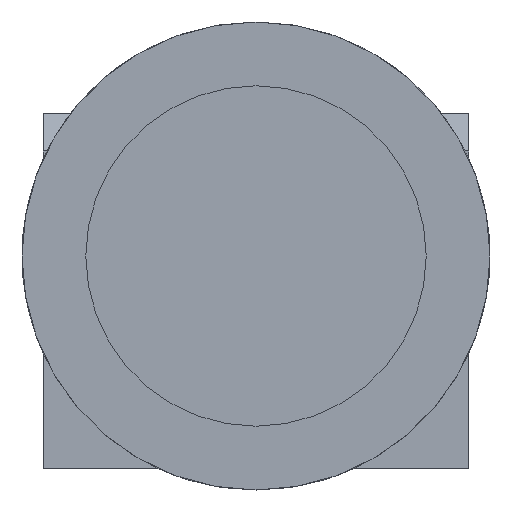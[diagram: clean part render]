
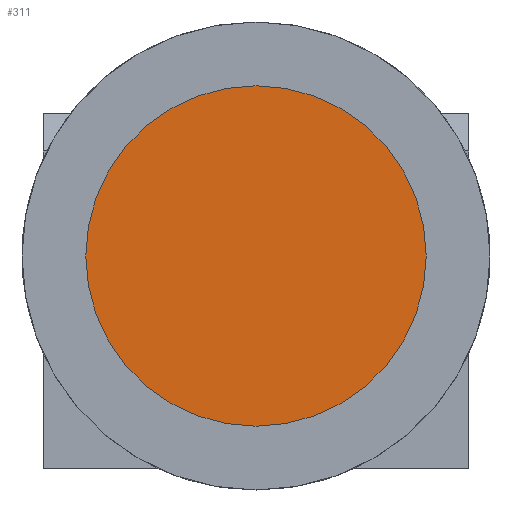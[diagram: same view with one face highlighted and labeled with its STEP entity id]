
A CAD part, front view. The second image highlights one B-rep face of the part: STEP entity #311.
In plain terms, the highlighted planar face has unit normal (0, -1, 0).
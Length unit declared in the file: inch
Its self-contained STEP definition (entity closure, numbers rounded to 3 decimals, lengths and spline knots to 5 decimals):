
#12 = AXIS2_PLACEMENT_3D ( 'NONE', #69, #70, #71 ) ;
#20 = FACE_OUTER_BOUND ( 'NONE', #1176, .T. ) ;
#68 = PLANE ( 'NONE',  #12 ) ;
#69 = CARTESIAN_POINT ( 'NONE',  ( 0.625, -0.533, 0. ) ) ;
#70 = DIRECTION ( 'NONE',  ( 0., -1., 0. ) ) ;
#71 = DIRECTION ( 'NONE',  ( 0., 0., -1. ) ) ;
#238 = EDGE_CURVE ( 'NONE', #942, #943, #383, .T. ) ;
#268 = EDGE_CURVE ( 'NONE', #943, #942, #393, .T. ) ;
#311 = ADVANCED_FACE ( 'NONE', ( #20 ), #68, .T. ) ;
#383 = CIRCLE ( 'NONE', #1828, 0.5 ) ;
#393 = CIRCLE ( 'NONE', #1805, 0.5 ) ;
#527 = CARTESIAN_POINT ( 'NONE',  ( 0.625, -0.533, -0.5 ) ) ;
#528 = CARTESIAN_POINT ( 'NONE',  ( 0.625, -0.533, 0.5 ) ) ;
#942 = VERTEX_POINT ( 'NONE', #527 ) ;
#943 = VERTEX_POINT ( 'NONE', #528 ) ;
#1050 = ORIENTED_EDGE ( 'NONE', *, *, #268, .F. ) ;
#1051 = ORIENTED_EDGE ( 'NONE', *, *, #238, .F. ) ;
#1176 = EDGE_LOOP ( 'NONE', ( #1050, #1051 ) ) ;
#1472 = CARTESIAN_POINT ( 'NONE',  ( 0.625, -0.533, 0. ) ) ;
#1473 = DIRECTION ( 'NONE',  ( 0., 1., 0. ) ) ;
#1474 = DIRECTION ( 'NONE',  ( 0., 0., 1. ) ) ;
#1573 = CARTESIAN_POINT ( 'NONE',  ( 0.625, -0.533, 0. ) ) ;
#1574 = DIRECTION ( 'NONE',  ( 0., 1., 0. ) ) ;
#1575 = DIRECTION ( 'NONE',  ( 0., 0., 1. ) ) ;
#1805 = AXIS2_PLACEMENT_3D ( 'NONE', #1573, #1574, #1575 ) ;
#1828 = AXIS2_PLACEMENT_3D ( 'NONE', #1472, #1473, #1474 ) ;
